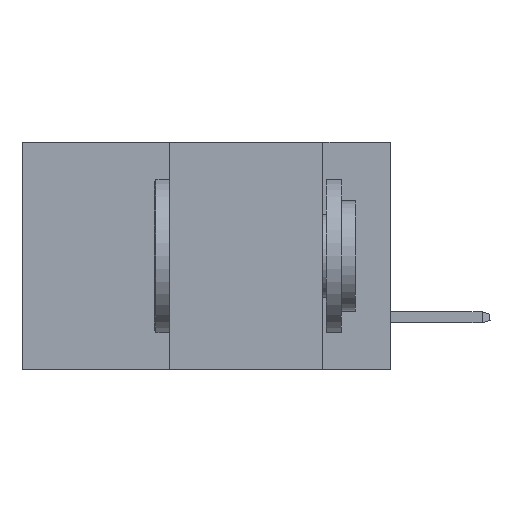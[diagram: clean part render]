
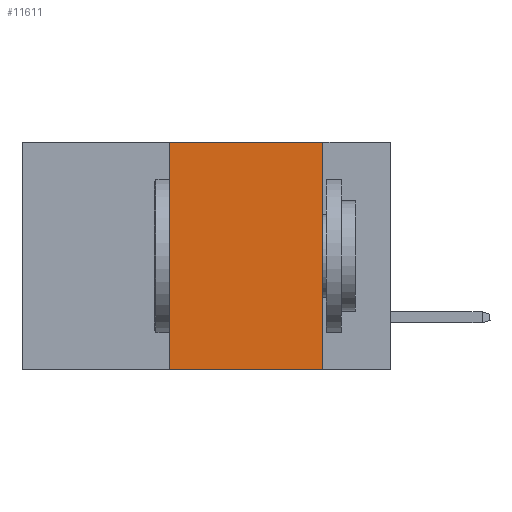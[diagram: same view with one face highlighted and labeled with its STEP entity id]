
A CAD part, left-side view. The second image highlights one B-rep face of the part: STEP entity #11611.
In plain terms, the highlighted planar face has unit normal (-1, 0, 0).
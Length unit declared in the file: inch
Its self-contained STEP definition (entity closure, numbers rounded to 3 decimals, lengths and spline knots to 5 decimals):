
#71 = CARTESIAN_POINT ( 'NONE',  ( 0., 0.6, 0. ) ) ;
#889 = EDGE_CURVE ( 'NONE', #15315, #36095, #7799, .T. ) ;
#2580 = EDGE_CURVE ( 'NONE', #9622, #15315, #25832, .T. ) ;
#3366 = ORIENTED_EDGE ( 'NONE', *, *, #22715, .F. ) ;
#6094 = DIRECTION ( 'NONE',  ( 0., -1., 0. ) ) ;
#7336 = CARTESIAN_POINT ( 'NONE',  ( 0., 0.6, -0.37 ) ) ;
#7453 = DIRECTION ( 'NONE',  ( 0., -1., 0. ) ) ;
#7530 = PLANE ( 'NONE',  #9704 ) ;
#7799 = LINE ( 'NONE', #19542, #16181 ) ;
#7999 = CARTESIAN_POINT ( 'NONE',  ( 0., 0.36, 0. ) ) ;
#9622 = VERTEX_POINT ( 'NONE', #7999 ) ;
#9704 = AXIS2_PLACEMENT_3D ( 'NONE', #10409, #25535, #22183 ) ;
#10409 = CARTESIAN_POINT ( 'NONE',  ( 0., 0.6, 0. ) ) ;
#11611 = ADVANCED_FACE ( 'NONE', ( #11642 ), #7530, .F. ) ;
#11642 = FACE_OUTER_BOUND ( 'NONE', #16442, .T. ) ;
#15315 = VERTEX_POINT ( 'NONE', #26148 ) ;
#16181 = VECTOR ( 'NONE', #22398, 39.37008 ) ;
#16442 = EDGE_LOOP ( 'NONE', ( #17223, #17453, #3366, #25354 ) ) ;
#17223 = ORIENTED_EDGE ( 'NONE', *, *, #889, .F. ) ;
#17228 = VECTOR ( 'NONE', #25769, 39.37008 ) ;
#17453 = ORIENTED_EDGE ( 'NONE', *, *, #2580, .F. ) ;
#17511 = VERTEX_POINT ( 'NONE', #24264 ) ;
#19542 = CARTESIAN_POINT ( 'NONE',  ( 0., 0.11, 0. ) ) ;
#19566 = LINE ( 'NONE', #7336, #31835 ) ;
#22183 = DIRECTION ( 'NONE',  ( 0., 0., -1. ) ) ;
#22398 = DIRECTION ( 'NONE',  ( 0., 0., -1. ) ) ;
#22715 = EDGE_CURVE ( 'NONE', #17511, #9622, #38170, .T. ) ;
#24264 = CARTESIAN_POINT ( 'NONE',  ( 0., 0.36, -0.37 ) ) ;
#25354 = ORIENTED_EDGE ( 'NONE', *, *, #37445, .T. ) ;
#25535 = DIRECTION ( 'NONE',  ( 1., 0., 0. ) ) ;
#25769 = DIRECTION ( 'NONE',  ( 0., 0., 1. ) ) ;
#25832 = LINE ( 'NONE', #71, #27686 ) ;
#26148 = CARTESIAN_POINT ( 'NONE',  ( 0., 0.11, 0. ) ) ;
#27686 = VECTOR ( 'NONE', #6094, 39.37008 ) ;
#31835 = VECTOR ( 'NONE', #7453, 39.37008 ) ;
#31955 = CARTESIAN_POINT ( 'NONE',  ( 0., 0.11, -0.37 ) ) ;
#36095 = VERTEX_POINT ( 'NONE', #31955 ) ;
#37445 = EDGE_CURVE ( 'NONE', #17511, #36095, #19566, .T. ) ;
#37493 = CARTESIAN_POINT ( 'NONE',  ( 0., 0.36, 0. ) ) ;
#38170 = LINE ( 'NONE', #37493, #17228 ) ;
